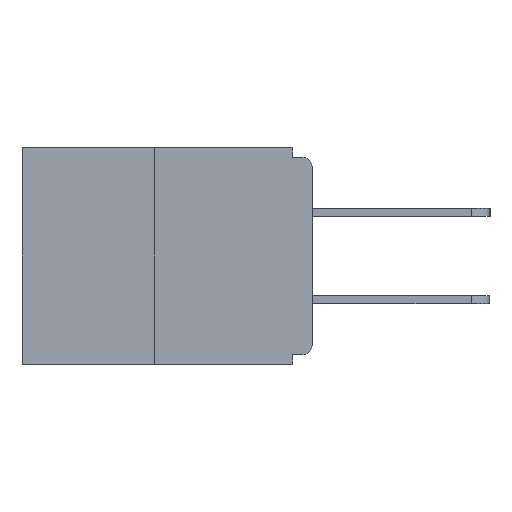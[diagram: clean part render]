
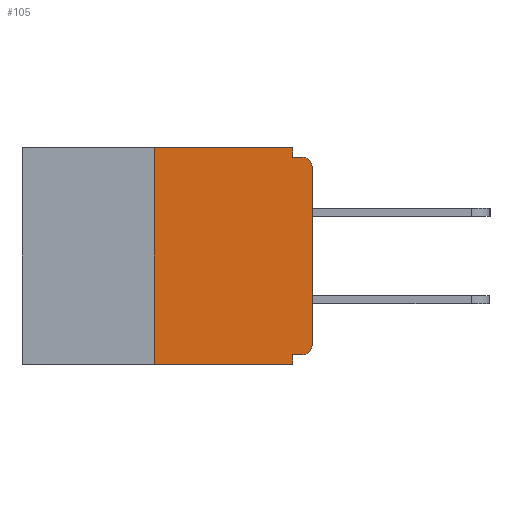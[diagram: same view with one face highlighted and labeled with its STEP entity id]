
A CAD part, left-side view. The second image highlights one B-rep face of the part: STEP entity #105.
In plain terms, the highlighted planar face has unit normal (-1, 0, 0).
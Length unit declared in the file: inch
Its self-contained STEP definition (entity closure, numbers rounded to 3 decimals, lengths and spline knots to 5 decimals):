
#105 = ADVANCED_FACE ( 'NONE', ( #6121 ), #1802, .F. ) ;
#271 = LINE ( 'NONE', #22594, #22735 ) ;
#579 = AXIS2_PLACEMENT_3D ( 'NONE', #9004, #6815, #26426 ) ;
#736 = CARTESIAN_POINT ( 'NONE',  ( 0., 0., -0.015 ) ) ;
#871 = CARTESIAN_POINT ( 'NONE',  ( 0., 0.015, -0.015 ) ) ;
#970 = VECTOR ( 'NONE', #19675, 39.37008 ) ;
#1095 = DIRECTION ( 'NONE',  ( 0., -1., 0. ) ) ;
#1802 = PLANE ( 'NONE',  #11179 ) ;
#1861 = ORIENTED_EDGE ( 'NONE', *, *, #8237, .F. ) ;
#2144 = LINE ( 'NONE', #24646, #15394 ) ;
#2230 = EDGE_CURVE ( 'NONE', #14984, #22250, #6756, .T. ) ;
#2329 = ORIENTED_EDGE ( 'NONE', *, *, #4323, .T. ) ;
#2340 = DIRECTION ( 'NONE',  ( 0., -1., 0. ) ) ;
#2794 = CARTESIAN_POINT ( 'NONE',  ( 0., 0.25, 0. ) ) ;
#3749 = EDGE_CURVE ( 'NONE', #19230, #11001, #25369, .T. ) ;
#3837 = CIRCLE ( 'NONE', #579, 0.015 ) ;
#4323 = EDGE_CURVE ( 'NONE', #4401, #12278, #14077, .T. ) ;
#4401 = VERTEX_POINT ( 'NONE', #24238 ) ;
#4586 = ORIENTED_EDGE ( 'NONE', *, *, #11812, .F. ) ;
#5990 = CARTESIAN_POINT ( 'NONE',  ( 0., 0.015, -0.328 ) ) ;
#6121 = FACE_OUTER_BOUND ( 'NONE', #7238, .T. ) ;
#6756 = LINE ( 'NONE', #22049, #970 ) ;
#6815 = DIRECTION ( 'NONE',  ( -1., 0., 0. ) ) ;
#7238 = EDGE_LOOP ( 'NONE', ( #14170, #20121, #26645, #23820, #1861, #23278, #2329, #26537, #4586, #24318 ) ) ;
#7288 = VECTOR ( 'NONE', #23561, 39.37008 ) ;
#7967 = CARTESIAN_POINT ( 'NONE',  ( 0., 0.25, 0. ) ) ;
#8237 = EDGE_CURVE ( 'NONE', #24092, #26172, #2144, .T. ) ;
#8350 = DIRECTION ( 'NONE',  ( 1., 0., 0. ) ) ;
#9004 = CARTESIAN_POINT ( 'NONE',  ( 0., 0.015, -0.313 ) ) ;
#9566 = VERTEX_POINT ( 'NONE', #871 ) ;
#10084 = CARTESIAN_POINT ( 'NONE',  ( 0., 0.015, -0.03 ) ) ;
#10744 = DIRECTION ( 'NONE',  ( 0., 0., -1. ) ) ;
#11001 = VERTEX_POINT ( 'NONE', #7967 ) ;
#11172 = CARTESIAN_POINT ( 'NONE',  ( 0., 0.031, -0.015 ) ) ;
#11179 = AXIS2_PLACEMENT_3D ( 'NONE', #21391, #8350, #10744 ) ;
#11200 = VERTEX_POINT ( 'NONE', #12300 ) ;
#11271 = DIRECTION ( 'NONE',  ( 0., 0., 1. ) ) ;
#11771 = EDGE_CURVE ( 'NONE', #19230, #11200, #271, .T. ) ;
#11812 = EDGE_CURVE ( 'NONE', #22250, #9566, #17942, .T. ) ;
#12278 = VERTEX_POINT ( 'NONE', #13366 ) ;
#12300 = CARTESIAN_POINT ( 'NONE',  ( 0., 0.031, -0.343 ) ) ;
#13148 = EDGE_CURVE ( 'NONE', #11001, #14984, #21605, .T. ) ;
#13366 = CARTESIAN_POINT ( 'NONE',  ( 0., 0., -0.03 ) ) ;
#14077 = LINE ( 'NONE', #25464, #7288 ) ;
#14170 = ORIENTED_EDGE ( 'NONE', *, *, #13148, .F. ) ;
#14981 = CARTESIAN_POINT ( 'NONE',  ( 0., 0.25, -0.343 ) ) ;
#14984 = VERTEX_POINT ( 'NONE', #27857 ) ;
#15394 = VECTOR ( 'NONE', #26847, 39.37008 ) ;
#15756 = AXIS2_PLACEMENT_3D ( 'NONE', #10084, #25227, #18836 ) ;
#15887 = LINE ( 'NONE', #26955, #22003 ) ;
#16020 = DIRECTION ( 'NONE',  ( 0., -1., 0. ) ) ;
#16234 = CARTESIAN_POINT ( 'NONE',  ( 0., 0.031, -0.328 ) ) ;
#17942 = LINE ( 'NONE', #736, #20330 ) ;
#18798 = EDGE_CURVE ( 'NONE', #26172, #11200, #15887, .T. ) ;
#18836 = DIRECTION ( 'NONE',  ( 0., 0., -1. ) ) ;
#19230 = VERTEX_POINT ( 'NONE', #14981 ) ;
#19675 = DIRECTION ( 'NONE',  ( 0., 0., -1. ) ) ;
#20121 = ORIENTED_EDGE ( 'NONE', *, *, #3749, .F. ) ;
#20330 = VECTOR ( 'NONE', #16020, 39.37008 ) ;
#21391 = CARTESIAN_POINT ( 'NONE',  ( 0., 0.46, 0. ) ) ;
#21605 = LINE ( 'NONE', #21817, #21927 ) ;
#21627 = EDGE_CURVE ( 'NONE', #24092, #4401, #3837, .T. ) ;
#21817 = CARTESIAN_POINT ( 'NONE',  ( 0., 0.46, 0. ) ) ;
#21927 = VECTOR ( 'NONE', #2340, 39.37008 ) ;
#22003 = VECTOR ( 'NONE', #24945, 39.37008 ) ;
#22049 = CARTESIAN_POINT ( 'NONE',  ( 0., 0.031, 0. ) ) ;
#22171 = CIRCLE ( 'NONE', #15756, 0.015 ) ;
#22250 = VERTEX_POINT ( 'NONE', #11172 ) ;
#22453 = EDGE_CURVE ( 'NONE', #12278, #9566, #22171, .T. ) ;
#22594 = CARTESIAN_POINT ( 'NONE',  ( 0., 0.46, -0.343 ) ) ;
#22735 = VECTOR ( 'NONE', #1095, 39.37008 ) ;
#23278 = ORIENTED_EDGE ( 'NONE', *, *, #21627, .T. ) ;
#23561 = DIRECTION ( 'NONE',  ( 0., 0., 1. ) ) ;
#23820 = ORIENTED_EDGE ( 'NONE', *, *, #18798, .F. ) ;
#24092 = VERTEX_POINT ( 'NONE', #5990 ) ;
#24238 = CARTESIAN_POINT ( 'NONE',  ( 0., 0., -0.313 ) ) ;
#24318 = ORIENTED_EDGE ( 'NONE', *, *, #2230, .F. ) ;
#24646 = CARTESIAN_POINT ( 'NONE',  ( 0., 0., -0.328 ) ) ;
#24945 = DIRECTION ( 'NONE',  ( 0., 0., -1. ) ) ;
#25227 = DIRECTION ( 'NONE',  ( -1., 0., 0. ) ) ;
#25369 = LINE ( 'NONE', #2794, #27074 ) ;
#25464 = CARTESIAN_POINT ( 'NONE',  ( 0., 0., 0. ) ) ;
#26172 = VERTEX_POINT ( 'NONE', #16234 ) ;
#26426 = DIRECTION ( 'NONE',  ( 0., 0., -1. ) ) ;
#26537 = ORIENTED_EDGE ( 'NONE', *, *, #22453, .T. ) ;
#26645 = ORIENTED_EDGE ( 'NONE', *, *, #11771, .T. ) ;
#26847 = DIRECTION ( 'NONE',  ( 0., 1., 0. ) ) ;
#26955 = CARTESIAN_POINT ( 'NONE',  ( 0., 0.031, -0.343 ) ) ;
#27074 = VECTOR ( 'NONE', #11271, 39.37008 ) ;
#27857 = CARTESIAN_POINT ( 'NONE',  ( 0., 0.031, 0. ) ) ;
